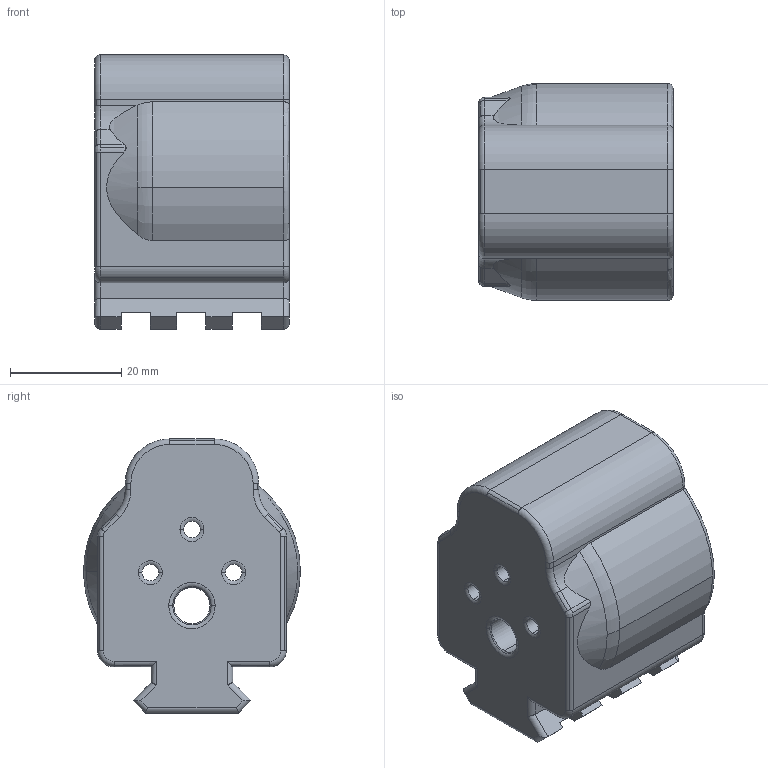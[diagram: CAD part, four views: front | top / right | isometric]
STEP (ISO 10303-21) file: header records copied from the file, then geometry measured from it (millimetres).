
FILE_DESCRIPTION (( 'STEP AP203' ), '1' );
FILE_NAME ('Brace_Adapter_ARBuffer.STEP', '2020-02-07T01:27:25', ( '' ), ( '' ), 'SwSTEP 2.0', 'SolidWorks 2019', '' );
FILE_SCHEMA (( 'CONFIG_CONTROL_DESIGN' ));
Length unit declared in the file: millimetre
Products named in the file (1): Brace_Adapter_ARBuffer
Bounding box: 35 x 38.99 x 49.32 mm (x, y, z)
Volume: 30279.4 mm3; surface area: 12990.4 mm2
Topology: 1 solids, 1 shells, 202 faces, 532 edges, 334 vertices
Faces by surface type: cylinder 99, plane 41, torus 29, cone 19, bspline 14
Entity records: 9756 total; most frequent: CARTESIAN_POINT 4959, ORIENTED_EDGE 1064, DIRECTION 938, EDGE_CURVE 532, AXIS2_PLACEMENT_3D 360, VERTEX_POINT 334, LINE 218, VECTOR 218
